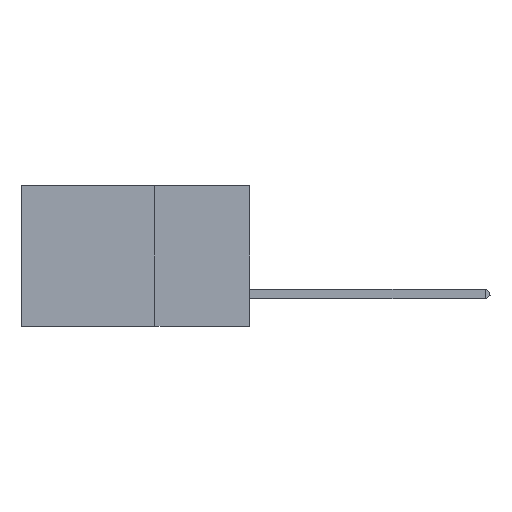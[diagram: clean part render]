
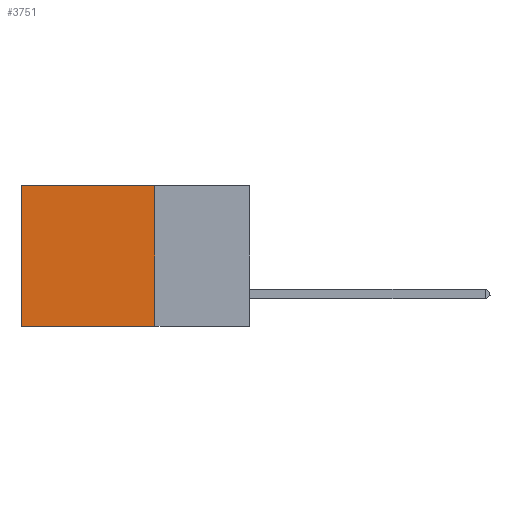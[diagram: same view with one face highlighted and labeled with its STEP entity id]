
A CAD part, left-side view. The second image highlights one B-rep face of the part: STEP entity #3751.
In plain terms, the highlighted planar face has unit normal (-1, 0, 0).
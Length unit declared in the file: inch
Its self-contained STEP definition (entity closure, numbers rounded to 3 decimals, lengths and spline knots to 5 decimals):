
#1165 = DIRECTION ( 'NONE',  ( 0., 1., 0. ) ) ;
#3162 = PLANE ( 'NONE',  #13957 ) ;
#3715 = ORIENTED_EDGE ( 'NONE', *, *, #6730, .T. ) ;
#3751 = ADVANCED_FACE ( 'NONE', ( #11403 ), #3162, .F. ) ;
#3849 = DIRECTION ( 'NONE',  ( 0., 0., -1. ) ) ;
#4684 = CARTESIAN_POINT ( 'NONE',  ( 0.2875, 0.25, 0. ) ) ;
#5144 = CARTESIAN_POINT ( 'NONE',  ( 0.2875, 0.25, 0. ) ) ;
#6341 = EDGE_CURVE ( 'NONE', #18854, #24244, #14621, .T. ) ;
#6730 = EDGE_CURVE ( 'NONE', #11936, #24244, #9103, .T. ) ;
#7100 = EDGE_CURVE ( 'NONE', #21792, #18854, #13670, .T. ) ;
#7124 = DIRECTION ( 'NONE',  ( 1., 0., 0. ) ) ;
#8792 = ORIENTED_EDGE ( 'NONE', *, *, #6341, .F. ) ;
#8999 = CARTESIAN_POINT ( 'NONE',  ( 0.2875, 0.6, 0. ) ) ;
#9016 = ORIENTED_EDGE ( 'NONE', *, *, #7100, .F. ) ;
#9103 = LINE ( 'NONE', #8999, #10319 ) ;
#10038 = EDGE_CURVE ( 'NONE', #21792, #11936, #10296, .T. ) ;
#10296 = LINE ( 'NONE', #15128, #13640 ) ;
#10319 = VECTOR ( 'NONE', #12688, 39.37008 ) ;
#11403 = FACE_OUTER_BOUND ( 'NONE', #23057, .T. ) ;
#11741 = CARTESIAN_POINT ( 'NONE',  ( 0.2875, 0.6, -0.37 ) ) ;
#11936 = VERTEX_POINT ( 'NONE', #20286 ) ;
#12624 = CARTESIAN_POINT ( 'NONE',  ( 0.2875, 0.25, -0.37 ) ) ;
#12688 = DIRECTION ( 'NONE',  ( 0., 0., -1. ) ) ;
#13054 = VECTOR ( 'NONE', #3849, 39.37008 ) ;
#13107 = DIRECTION ( 'NONE',  ( 0., 0., -1. ) ) ;
#13640 = VECTOR ( 'NONE', #1165, 39.37008 ) ;
#13670 = LINE ( 'NONE', #15488, #13054 ) ;
#13957 = AXIS2_PLACEMENT_3D ( 'NONE', #5144, #7124, #13107 ) ;
#14588 = DIRECTION ( 'NONE',  ( 0., 1., 0. ) ) ;
#14621 = LINE ( 'NONE', #12624, #17996 ) ;
#15128 = CARTESIAN_POINT ( 'NONE',  ( 0.2875, 0.25, 0. ) ) ;
#15488 = CARTESIAN_POINT ( 'NONE',  ( 0.2875, 0.25, 0. ) ) ;
#16890 = CARTESIAN_POINT ( 'NONE',  ( 0.2875, 0.25, -0.37 ) ) ;
#17996 = VECTOR ( 'NONE', #14588, 39.37008 ) ;
#18854 = VERTEX_POINT ( 'NONE', #16890 ) ;
#20286 = CARTESIAN_POINT ( 'NONE',  ( 0.2875, 0.6, 0. ) ) ;
#21762 = ORIENTED_EDGE ( 'NONE', *, *, #10038, .T. ) ;
#21792 = VERTEX_POINT ( 'NONE', #4684 ) ;
#23057 = EDGE_LOOP ( 'NONE', ( #3715, #8792, #9016, #21762 ) ) ;
#24244 = VERTEX_POINT ( 'NONE', #11741 ) ;
